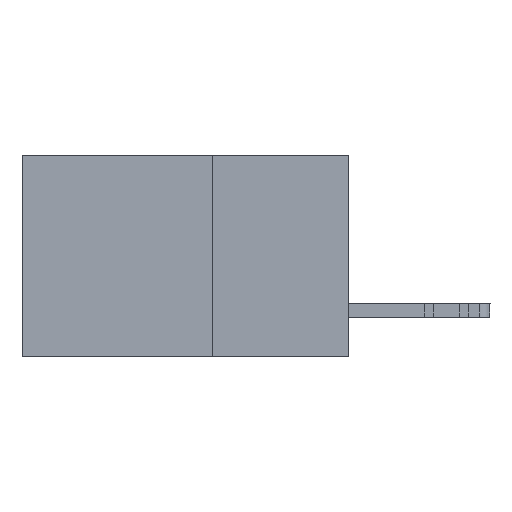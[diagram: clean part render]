
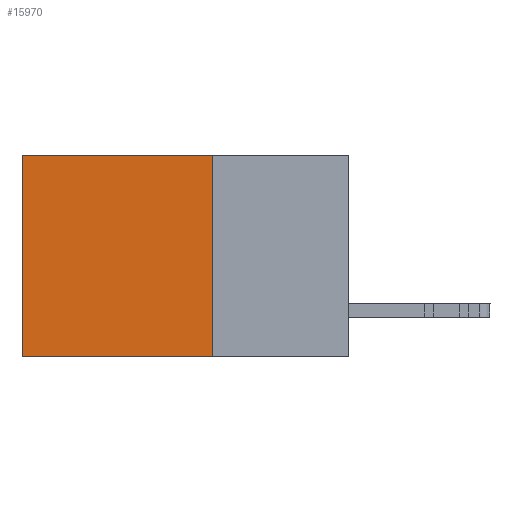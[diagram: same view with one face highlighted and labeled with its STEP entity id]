
A CAD part, left-side view. The second image highlights one B-rep face of the part: STEP entity #15970.
In plain terms, the highlighted planar face has unit normal (-1, 0, 0).
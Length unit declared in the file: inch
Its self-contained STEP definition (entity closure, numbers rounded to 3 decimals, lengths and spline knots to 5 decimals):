
#580 = DIRECTION ( 'NONE',  ( 0., 0., -1. ) ) ;
#924 = VERTEX_POINT ( 'NONE', #25016 ) ;
#1848 = AXIS2_PLACEMENT_3D ( 'NONE', #12404, #21831, #580 ) ;
#2030 = VECTOR ( 'NONE', #16315, 39.37008 ) ;
#2629 = EDGE_CURVE ( 'NONE', #15271, #8988, #3214, .T. ) ;
#2703 = LINE ( 'NONE', #8442, #2030 ) ;
#3214 = LINE ( 'NONE', #4914, #11477 ) ;
#4914 = CARTESIAN_POINT ( 'NONE',  ( 0.2615, 0.25, -0.37 ) ) ;
#5509 = LINE ( 'NONE', #13419, #15892 ) ;
#6380 = EDGE_CURVE ( 'NONE', #924, #8988, #13766, .T. ) ;
#7318 = ORIENTED_EDGE ( 'NONE', *, *, #14547, .T. ) ;
#7810 = EDGE_LOOP ( 'NONE', ( #22327, #15344, #22983, #7318 ) ) ;
#7878 = VECTOR ( 'NONE', #15450, 39.37008 ) ;
#8210 = EDGE_CURVE ( 'NONE', #17642, #15271, #2703, .T. ) ;
#8442 = CARTESIAN_POINT ( 'NONE',  ( 0.2615, 0.25, -0.37 ) ) ;
#8988 = VERTEX_POINT ( 'NONE', #9552 ) ;
#9552 = CARTESIAN_POINT ( 'NONE',  ( 0.2615, 0.6, -0.37 ) ) ;
#9706 = FACE_OUTER_BOUND ( 'NONE', #7810, .T. ) ;
#11343 = CARTESIAN_POINT ( 'NONE',  ( 0.2615, 0.25, 0. ) ) ;
#11477 = VECTOR ( 'NONE', #12827, 39.37008 ) ;
#12093 = CARTESIAN_POINT ( 'NONE',  ( 0.2615, 0.25, -0.37 ) ) ;
#12404 = CARTESIAN_POINT ( 'NONE',  ( 0.2615, 0.25, -0.37 ) ) ;
#12827 = DIRECTION ( 'NONE',  ( 0., 1., 0. ) ) ;
#13419 = CARTESIAN_POINT ( 'NONE',  ( 0.2615, 0.25, 0. ) ) ;
#13766 = LINE ( 'NONE', #17507, #7878 ) ;
#14547 = EDGE_CURVE ( 'NONE', #17642, #924, #5509, .T. ) ;
#15271 = VERTEX_POINT ( 'NONE', #12093 ) ;
#15344 = ORIENTED_EDGE ( 'NONE', *, *, #2629, .F. ) ;
#15450 = DIRECTION ( 'NONE',  ( 0., 0., -1. ) ) ;
#15892 = VECTOR ( 'NONE', #21280, 39.37008 ) ;
#15970 = ADVANCED_FACE ( 'NONE', ( #9706 ), #17575, .F. ) ;
#16315 = DIRECTION ( 'NONE',  ( 0., 0., -1. ) ) ;
#17507 = CARTESIAN_POINT ( 'NONE',  ( 0.2615, 0.6, -0.37 ) ) ;
#17575 = PLANE ( 'NONE',  #1848 ) ;
#17642 = VERTEX_POINT ( 'NONE', #11343 ) ;
#21280 = DIRECTION ( 'NONE',  ( 0., 1., 0. ) ) ;
#21831 = DIRECTION ( 'NONE',  ( 1., 0., 0. ) ) ;
#22327 = ORIENTED_EDGE ( 'NONE', *, *, #6380, .T. ) ;
#22983 = ORIENTED_EDGE ( 'NONE', *, *, #8210, .F. ) ;
#25016 = CARTESIAN_POINT ( 'NONE',  ( 0.2615, 0.6, 0. ) ) ;
